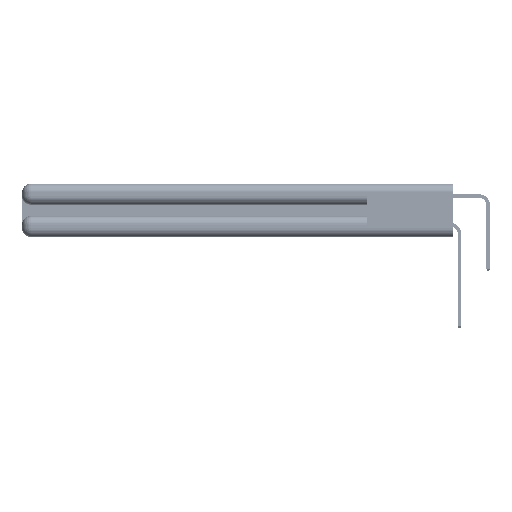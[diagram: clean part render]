
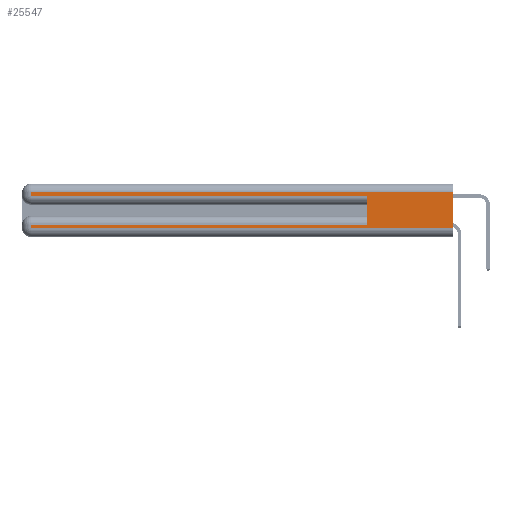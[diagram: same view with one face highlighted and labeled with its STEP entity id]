
A CAD part, left-side view. The second image highlights one B-rep face of the part: STEP entity #25547.
In plain terms, the highlighted planar face has unit normal (-1, 0, 0).
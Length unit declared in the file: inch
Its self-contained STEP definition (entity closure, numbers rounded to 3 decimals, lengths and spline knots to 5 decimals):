
#1094 = CARTESIAN_POINT ( 'NONE',  ( 0., 0.6, 0.145 ) ) ;
#1694 = CARTESIAN_POINT ( 'NONE',  ( 0., 2.94, 0.085 ) ) ;
#1866 = VECTOR ( 'NONE', #18907, 39.37008 ) ;
#5064 = ORIENTED_EDGE ( 'NONE', *, *, #5508, .F. ) ;
#5508 = EDGE_CURVE ( 'NONE', #6251, #22134, #30669, .T. ) ;
#6240 = VECTOR ( 'NONE', #18489, 39.37008 ) ;
#6251 = VERTEX_POINT ( 'NONE', #48512 ) ;
#6264 = VECTOR ( 'NONE', #33153, 39.37008 ) ;
#7544 = DIRECTION ( 'NONE',  ( 0., 0., -1. ) ) ;
#8387 = AXIS2_PLACEMENT_3D ( 'NONE', #15973, #33118, #7544 ) ;
#8525 = FACE_OUTER_BOUND ( 'NONE', #18901, .T. ) ;
#8694 = EDGE_CURVE ( 'NONE', #22852, #10404, #40300, .T. ) ;
#10200 = CARTESIAN_POINT ( 'NONE',  ( 0., 2.94, 0.37 ) ) ;
#10320 = CARTESIAN_POINT ( 'NONE',  ( 0., 2.94, 0.31 ) ) ;
#10404 = VERTEX_POINT ( 'NONE', #32003 ) ;
#11669 = VERTEX_POINT ( 'NONE', #36727 ) ;
#11701 = VERTEX_POINT ( 'NONE', #28529 ) ;
#14934 = LINE ( 'NONE', #39715, #6240 ) ;
#15973 = CARTESIAN_POINT ( 'NONE',  ( 0., 0., 0.37 ) ) ;
#18489 = DIRECTION ( 'NONE',  ( 0., 1., 0. ) ) ;
#18901 = EDGE_LOOP ( 'NONE', ( #51060, #40400, #20408, #49780, #5064, #24501, #28496, #32498 ) ) ;
#18907 = DIRECTION ( 'NONE',  ( 0., -1., 0. ) ) ;
#19838 = EDGE_CURVE ( 'NONE', #11701, #22134, #21233, .T. ) ;
#20408 = ORIENTED_EDGE ( 'NONE', *, *, #36975, .T. ) ;
#21233 = LINE ( 'NONE', #40618, #53933 ) ;
#22134 = VERTEX_POINT ( 'NONE', #31305 ) ;
#22852 = VERTEX_POINT ( 'NONE', #1694 ) ;
#24501 = ORIENTED_EDGE ( 'NONE', *, *, #53411, .T. ) ;
#24847 = VECTOR ( 'NONE', #30620, 39.37008 ) ;
#25547 = ADVANCED_FACE ( 'NONE', ( #8525 ), #28835, .F. ) ;
#25947 = VECTOR ( 'NONE', #40027, 39.37008 ) ;
#26791 = DIRECTION ( 'NONE',  ( 0., 0., 1. ) ) ;
#27725 = VERTEX_POINT ( 'NONE', #10320 ) ;
#28496 = ORIENTED_EDGE ( 'NONE', *, *, #8694, .T. ) ;
#28529 = CARTESIAN_POINT ( 'NONE',  ( 0., 2.94, 0.285 ) ) ;
#28835 = PLANE ( 'NONE',  #8387 ) ;
#30259 = LINE ( 'NONE', #37922, #40262 ) ;
#30620 = DIRECTION ( 'NONE',  ( 0., 0., -1. ) ) ;
#30669 = LINE ( 'NONE', #1094, #39340 ) ;
#31305 = CARTESIAN_POINT ( 'NONE',  ( 0., 0.6, 0.285 ) ) ;
#32003 = CARTESIAN_POINT ( 'NONE',  ( 0., 2.94, 0.06 ) ) ;
#32498 = ORIENTED_EDGE ( 'NONE', *, *, #36592, .T. ) ;
#33118 = DIRECTION ( 'NONE',  ( 1., 0., 0. ) ) ;
#33153 = DIRECTION ( 'NONE',  ( 0., 0., -1. ) ) ;
#36173 = LINE ( 'NONE', #51877, #24847 ) ;
#36350 = DIRECTION ( 'NONE',  ( 0., -1., 0. ) ) ;
#36592 = EDGE_CURVE ( 'NONE', #10404, #46799, #47316, .T. ) ;
#36727 = CARTESIAN_POINT ( 'NONE',  ( 0., 0., 0.31 ) ) ;
#36975 = EDGE_CURVE ( 'NONE', #27725, #11701, #37262, .T. ) ;
#37262 = LINE ( 'NONE', #10200, #25947 ) ;
#37922 = CARTESIAN_POINT ( 'NONE',  ( 0., 0., 0.085 ) ) ;
#39340 = VECTOR ( 'NONE', #26791, 39.37008 ) ;
#39715 = CARTESIAN_POINT ( 'NONE',  ( 0., 0., 0.31 ) ) ;
#40027 = DIRECTION ( 'NONE',  ( 0., 0., -1. ) ) ;
#40131 = CARTESIAN_POINT ( 'NONE',  ( 0., 0., 0.06 ) ) ;
#40262 = VECTOR ( 'NONE', #42198, 39.37008 ) ;
#40300 = LINE ( 'NONE', #54412, #6264 ) ;
#40400 = ORIENTED_EDGE ( 'NONE', *, *, #54145, .T. ) ;
#40618 = CARTESIAN_POINT ( 'NONE',  ( 0., 0., 0.285 ) ) ;
#41610 = EDGE_CURVE ( 'NONE', #11669, #46799, #36173, .T. ) ;
#42198 = DIRECTION ( 'NONE',  ( 0., 1., 0. ) ) ;
#46799 = VERTEX_POINT ( 'NONE', #47342 ) ;
#47316 = LINE ( 'NONE', #40131, #1866 ) ;
#47342 = CARTESIAN_POINT ( 'NONE',  ( 0., 0., 0.06 ) ) ;
#48512 = CARTESIAN_POINT ( 'NONE',  ( 0., 0.6, 0.085 ) ) ;
#49780 = ORIENTED_EDGE ( 'NONE', *, *, #19838, .T. ) ;
#51060 = ORIENTED_EDGE ( 'NONE', *, *, #41610, .F. ) ;
#51877 = CARTESIAN_POINT ( 'NONE',  ( 0., 0., 0.37 ) ) ;
#53411 = EDGE_CURVE ( 'NONE', #6251, #22852, #30259, .T. ) ;
#53933 = VECTOR ( 'NONE', #36350, 39.37008 ) ;
#54145 = EDGE_CURVE ( 'NONE', #11669, #27725, #14934, .T. ) ;
#54412 = CARTESIAN_POINT ( 'NONE',  ( 0., 2.94, 0.37 ) ) ;
